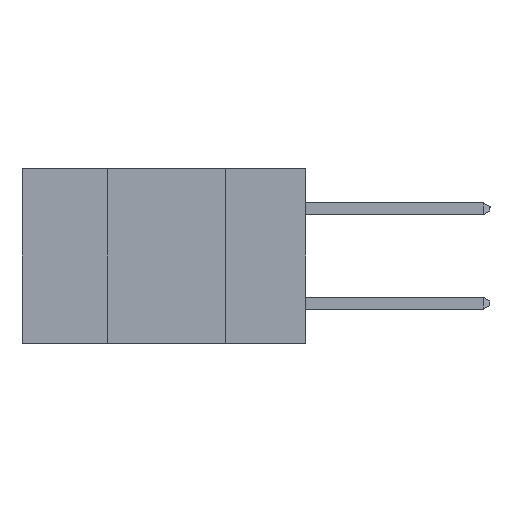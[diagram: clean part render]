
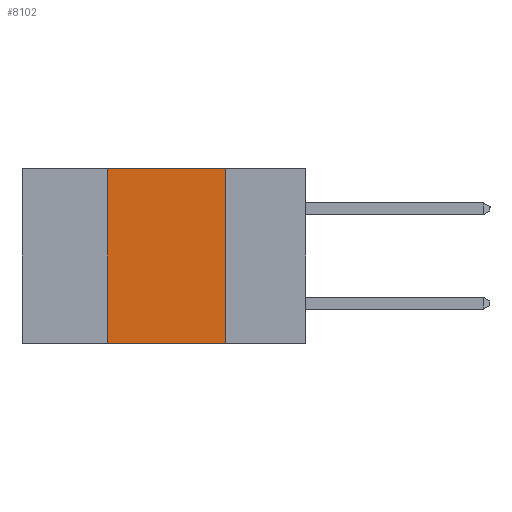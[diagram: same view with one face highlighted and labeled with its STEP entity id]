
A CAD part, left-side view. The second image highlights one B-rep face of the part: STEP entity #8102.
In plain terms, the highlighted planar face has unit normal (-1, 0, 0).
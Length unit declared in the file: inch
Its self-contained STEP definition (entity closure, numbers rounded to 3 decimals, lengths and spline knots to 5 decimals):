
#656 = EDGE_CURVE ( 'NONE', #15977, #5138, #8941, .T. ) ;
#812 = CARTESIAN_POINT ( 'NONE',  ( 0., 0.42, -0.37 ) ) ;
#1207 = VERTEX_POINT ( 'NONE', #6590 ) ;
#1232 = VERTEX_POINT ( 'NONE', #14425 ) ;
#2265 = DIRECTION ( 'NONE',  ( 0., -1., 0. ) ) ;
#3007 = VECTOR ( 'NONE', #15608, 39.37008 ) ;
#3602 = VECTOR ( 'NONE', #12709, 39.37008 ) ;
#3625 = CARTESIAN_POINT ( 'NONE',  ( 0., 0.42, 0. ) ) ;
#3664 = ORIENTED_EDGE ( 'NONE', *, *, #656, .F. ) ;
#4633 = PLANE ( 'NONE',  #15471 ) ;
#5110 = LINE ( 'NONE', #9397, #9273 ) ;
#5138 = VERTEX_POINT ( 'NONE', #3625 ) ;
#5164 = ORIENTED_EDGE ( 'NONE', *, *, #11617, .F. ) ;
#5873 = DIRECTION ( 'NONE',  ( 0., 0., -1. ) ) ;
#6590 = CARTESIAN_POINT ( 'NONE',  ( 0., 0.17, 0. ) ) ;
#7288 = CARTESIAN_POINT ( 'NONE',  ( 0., 0.6, -0.37 ) ) ;
#7345 = EDGE_LOOP ( 'NONE', ( #5164, #9193, #3664, #17350 ) ) ;
#7634 = LINE ( 'NONE', #15738, #14111 ) ;
#7691 = DIRECTION ( 'NONE',  ( 0., 0., -1. ) ) ;
#8102 = ADVANCED_FACE ( 'NONE', ( #8738 ), #4633, .F. ) ;
#8738 = FACE_OUTER_BOUND ( 'NONE', #7345, .T. ) ;
#8941 = LINE ( 'NONE', #812, #3007 ) ;
#9193 = ORIENTED_EDGE ( 'NONE', *, *, #12976, .F. ) ;
#9273 = VECTOR ( 'NONE', #7691, 39.37008 ) ;
#9397 = CARTESIAN_POINT ( 'NONE',  ( 0., 0.17, -0.37 ) ) ;
#11617 = EDGE_CURVE ( 'NONE', #1207, #1232, #5110, .T. ) ;
#12709 = DIRECTION ( 'NONE',  ( 0., -1., 0. ) ) ;
#12976 = EDGE_CURVE ( 'NONE', #5138, #1207, #7634, .T. ) ;
#14111 = VECTOR ( 'NONE', #2265, 39.37008 ) ;
#14135 = LINE ( 'NONE', #7288, #3602 ) ;
#14425 = CARTESIAN_POINT ( 'NONE',  ( 0., 0.17, -0.37 ) ) ;
#15457 = CARTESIAN_POINT ( 'NONE',  ( 0., 0.42, -0.37 ) ) ;
#15471 = AXIS2_PLACEMENT_3D ( 'NONE', #15582, #16648, #5873 ) ;
#15582 = CARTESIAN_POINT ( 'NONE',  ( 0., 0.6, 0. ) ) ;
#15597 = EDGE_CURVE ( 'NONE', #15977, #1232, #14135, .T. ) ;
#15608 = DIRECTION ( 'NONE',  ( 0., 0., 1. ) ) ;
#15738 = CARTESIAN_POINT ( 'NONE',  ( 0., 0.6, 0. ) ) ;
#15977 = VERTEX_POINT ( 'NONE', #15457 ) ;
#16648 = DIRECTION ( 'NONE',  ( 1., 0., 0. ) ) ;
#17350 = ORIENTED_EDGE ( 'NONE', *, *, #15597, .T. ) ;
